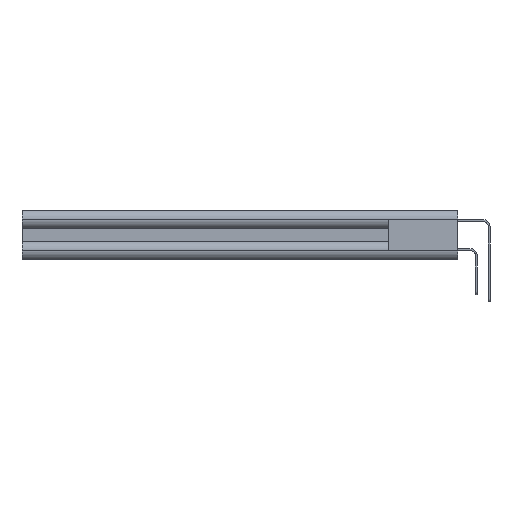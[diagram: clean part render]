
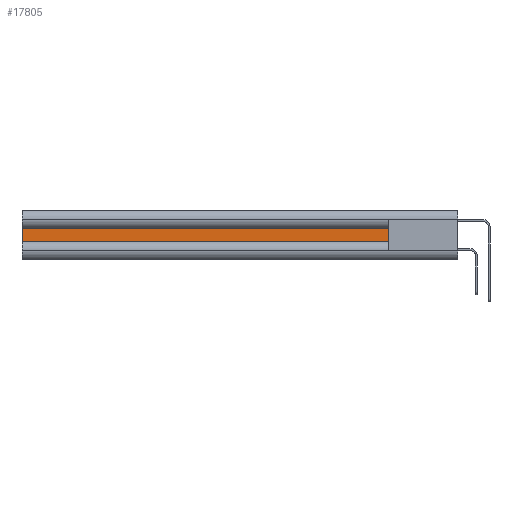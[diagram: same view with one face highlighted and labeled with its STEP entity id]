
A CAD part, left-side view. The second image highlights one B-rep face of the part: STEP entity #17805.
In plain terms, the highlighted planar face has unit normal (-1, 0, 0).
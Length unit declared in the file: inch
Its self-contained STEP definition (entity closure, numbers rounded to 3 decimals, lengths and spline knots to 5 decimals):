
#2519 = VECTOR ( 'NONE', #9807, 39.37008 ) ;
#2701 = CARTESIAN_POINT ( 'NONE',  ( 0.044, 3., -0.0465 ) ) ;
#2878 = CARTESIAN_POINT ( 'NONE',  ( 0.044, 0.473, -0.0465 ) ) ;
#2882 = EDGE_LOOP ( 'NONE', ( #4153, #12332, #10355, #20564 ) ) ;
#2922 = VERTEX_POINT ( 'NONE', #18774 ) ;
#2954 = EDGE_CURVE ( 'NONE', #14372, #8829, #19622, .T. ) ;
#3466 = VECTOR ( 'NONE', #20874, 39.37008 ) ;
#4153 = ORIENTED_EDGE ( 'NONE', *, *, #5352, .T. ) ;
#4465 = CARTESIAN_POINT ( 'NONE',  ( 0.044, 3., -0.0465 ) ) ;
#5352 = EDGE_CURVE ( 'NONE', #2922, #14372, #8339, .T. ) ;
#6117 = CARTESIAN_POINT ( 'NONE',  ( 0.044, 0.37012, -0.0465 ) ) ;
#7140 = AXIS2_PLACEMENT_3D ( 'NONE', #20285, #9619, #22033 ) ;
#7518 = EDGE_CURVE ( 'NONE', #19894, #8829, #16952, .T. ) ;
#8135 = DIRECTION ( 'NONE',  ( 0., 0., -1. ) ) ;
#8339 = LINE ( 'NONE', #22526, #3466 ) ;
#8559 = VECTOR ( 'NONE', #11714, 39.37008 ) ;
#8829 = VERTEX_POINT ( 'NONE', #2701 ) ;
#9541 = PLANE ( 'NONE',  #7140 ) ;
#9619 = DIRECTION ( 'NONE',  ( 1., 0., 0. ) ) ;
#9807 = DIRECTION ( 'NONE',  ( 0., 1., 0. ) ) ;
#9891 = CARTESIAN_POINT ( 'NONE',  ( 0.044, 0.473, -0.0465 ) ) ;
#10355 = ORIENTED_EDGE ( 'NONE', *, *, #7518, .F. ) ;
#11714 = DIRECTION ( 'NONE',  ( 0., 0., -1. ) ) ;
#12332 = ORIENTED_EDGE ( 'NONE', *, *, #2954, .T. ) ;
#12336 = EDGE_CURVE ( 'NONE', #2922, #19894, #22718, .T. ) ;
#14372 = VERTEX_POINT ( 'NONE', #14512 ) ;
#14512 = CARTESIAN_POINT ( 'NONE',  ( 0.044, 3., 0.0465 ) ) ;
#16952 = LINE ( 'NONE', #6117, #2519 ) ;
#17805 = ADVANCED_FACE ( 'NONE', ( #20248 ), #9541, .F. ) ;
#18774 = CARTESIAN_POINT ( 'NONE',  ( 0.044, 0.473, 0.0465 ) ) ;
#19622 = LINE ( 'NONE', #4465, #23145 ) ;
#19894 = VERTEX_POINT ( 'NONE', #2878 ) ;
#20248 = FACE_OUTER_BOUND ( 'NONE', #2882, .T. ) ;
#20285 = CARTESIAN_POINT ( 'NONE',  ( 0.044, 0.37012, -0.0465 ) ) ;
#20564 = ORIENTED_EDGE ( 'NONE', *, *, #12336, .F. ) ;
#20874 = DIRECTION ( 'NONE',  ( 0., 1., 0. ) ) ;
#22033 = DIRECTION ( 'NONE',  ( 0., 0., -1. ) ) ;
#22526 = CARTESIAN_POINT ( 'NONE',  ( 0.044, 0.37012, 0.0465 ) ) ;
#22718 = LINE ( 'NONE', #9891, #8559 ) ;
#23145 = VECTOR ( 'NONE', #8135, 39.37008 ) ;
